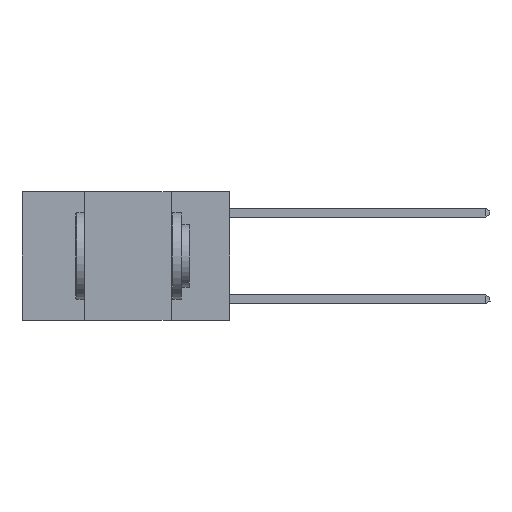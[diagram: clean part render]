
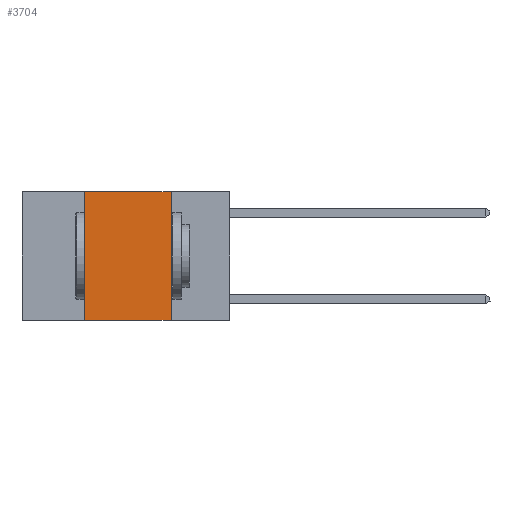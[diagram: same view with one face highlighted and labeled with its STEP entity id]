
A CAD part, left-side view. The second image highlights one B-rep face of the part: STEP entity #3704.
In plain terms, the highlighted planar face has unit normal (-1, 0, 0).
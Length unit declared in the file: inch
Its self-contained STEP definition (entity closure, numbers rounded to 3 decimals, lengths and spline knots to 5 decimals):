
#314 = CARTESIAN_POINT ( 'NONE',  ( 0., 0.42, 0. ) ) ;
#622 = LINE ( 'NONE', #10191, #5532 ) ;
#1038 = CARTESIAN_POINT ( 'NONE',  ( 0., 0.6, 0. ) ) ;
#1443 = VERTEX_POINT ( 'NONE', #2226 ) ;
#1745 = VECTOR ( 'NONE', #6906, 39.37008 ) ;
#1969 = VERTEX_POINT ( 'NONE', #314 ) ;
#2058 = AXIS2_PLACEMENT_3D ( 'NONE', #8641, #3048, #9562 ) ;
#2076 = LINE ( 'NONE', #1038, #1745 ) ;
#2226 = CARTESIAN_POINT ( 'NONE',  ( 0., 0.42, -0.37 ) ) ;
#2818 = ORIENTED_EDGE ( 'NONE', *, *, #8311, .F. ) ;
#2929 = EDGE_CURVE ( 'NONE', #1443, #1969, #3128, .T. ) ;
#2933 = CARTESIAN_POINT ( 'NONE',  ( 0., 0.42, 0. ) ) ;
#3048 = DIRECTION ( 'NONE',  ( 1., 0., 0. ) ) ;
#3128 = LINE ( 'NONE', #2933, #10228 ) ;
#3322 = ORIENTED_EDGE ( 'NONE', *, *, #7460, .F. ) ;
#3704 = ADVANCED_FACE ( 'NONE', ( #9799 ), #10412, .F. ) ;
#4089 = ORIENTED_EDGE ( 'NONE', *, *, #2929, .F. ) ;
#4141 = ORIENTED_EDGE ( 'NONE', *, *, #9305, .T. ) ;
#5229 = CARTESIAN_POINT ( 'NONE',  ( 0., 0.17, -0.37 ) ) ;
#5243 = VERTEX_POINT ( 'NONE', #5439 ) ;
#5439 = CARTESIAN_POINT ( 'NONE',  ( 0., 0.17, 0. ) ) ;
#5532 = VECTOR ( 'NONE', #11104, 39.37008 ) ;
#6166 = CARTESIAN_POINT ( 'NONE',  ( 0., 0.17, 0. ) ) ;
#6860 = VECTOR ( 'NONE', #11611, 39.37008 ) ;
#6906 = DIRECTION ( 'NONE',  ( 0., -1., 0. ) ) ;
#7460 = EDGE_CURVE ( 'NONE', #1969, #5243, #2076, .T. ) ;
#7729 = LINE ( 'NONE', #6166, #6860 ) ;
#8311 = EDGE_CURVE ( 'NONE', #5243, #10313, #7729, .T. ) ;
#8641 = CARTESIAN_POINT ( 'NONE',  ( 0., 0.6, 0. ) ) ;
#9305 = EDGE_CURVE ( 'NONE', #1443, #10313, #622, .T. ) ;
#9562 = DIRECTION ( 'NONE',  ( 0., 0., -1. ) ) ;
#9799 = FACE_OUTER_BOUND ( 'NONE', #11716, .T. ) ;
#10191 = CARTESIAN_POINT ( 'NONE',  ( 0., 0.6, -0.37 ) ) ;
#10228 = VECTOR ( 'NONE', #12122, 39.37008 ) ;
#10313 = VERTEX_POINT ( 'NONE', #5229 ) ;
#10412 = PLANE ( 'NONE',  #2058 ) ;
#11104 = DIRECTION ( 'NONE',  ( 0., -1., 0. ) ) ;
#11611 = DIRECTION ( 'NONE',  ( 0., 0., -1. ) ) ;
#11716 = EDGE_LOOP ( 'NONE', ( #2818, #3322, #4089, #4141 ) ) ;
#12122 = DIRECTION ( 'NONE',  ( 0., 0., 1. ) ) ;
